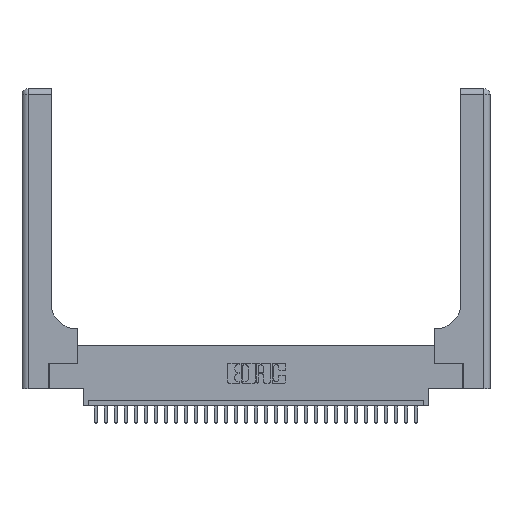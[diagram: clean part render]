
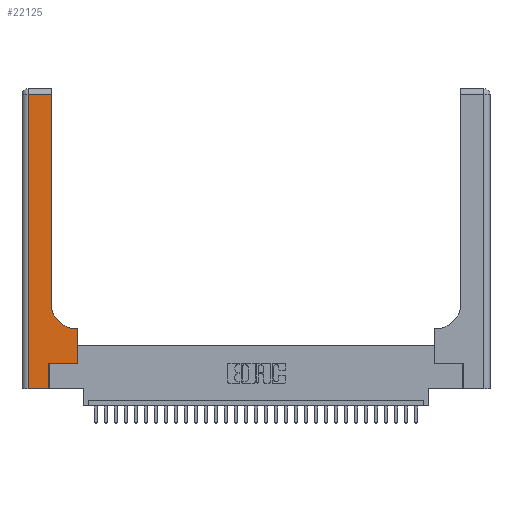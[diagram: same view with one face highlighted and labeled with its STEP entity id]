
A CAD part, top view. The second image highlights one B-rep face of the part: STEP entity #22125.
In plain terms, the highlighted planar face has unit normal (0, 0, 1).
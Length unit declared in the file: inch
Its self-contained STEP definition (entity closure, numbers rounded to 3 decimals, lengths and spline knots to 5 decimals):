
#57 = CARTESIAN_POINT ( 'NONE',  ( 0.269, 0.25, 0.37 ) ) ;
#70 = ORIENTED_EDGE ( 'NONE', *, *, #18516, .T. ) ;
#217 = DIRECTION ( 'NONE',  ( -1., 0., 0. ) ) ;
#860 = EDGE_CURVE ( 'NONE', #13966, #17433, #23793, .T. ) ;
#1548 = DIRECTION ( 'NONE',  ( 0., 1., 0. ) ) ;
#1826 = CARTESIAN_POINT ( 'NONE',  ( 0.5585, 0.6, 0.37 ) ) ;
#3278 = CARTESIAN_POINT ( 'NONE',  ( 0.2915, 0.85, 0.37 ) ) ;
#3948 = CARTESIAN_POINT ( 'NONE',  ( 0.5585, 0.25, 0.37 ) ) ;
#4366 = DIRECTION ( 'NONE',  ( 0., 1., 0. ) ) ;
#5008 = DIRECTION ( 'NONE',  ( 1., 0., 0. ) ) ;
#5168 = DIRECTION ( 'NONE',  ( 1., 0., 0. ) ) ;
#5256 = CARTESIAN_POINT ( 'NONE',  ( 0.2915, 0.6, 0.37 ) ) ;
#5613 = EDGE_LOOP ( 'NONE', ( #27200, #24012, #6091, #30341, #8297, #6652, #70, #12628, #13001 ) ) ;
#5722 = VERTEX_POINT ( 'NONE', #7020 ) ;
#6091 = ORIENTED_EDGE ( 'NONE', *, *, #7182, .T. ) ;
#6527 = VECTOR ( 'NONE', #7818, 39.37008 ) ;
#6652 = ORIENTED_EDGE ( 'NONE', *, *, #8832, .T. ) ;
#7020 = CARTESIAN_POINT ( 'NONE',  ( 0.2915, 2.94, 0.37 ) ) ;
#7182 = EDGE_CURVE ( 'NONE', #18581, #13966, #21991, .T. ) ;
#7818 = DIRECTION ( 'NONE',  ( -1., 0., 0. ) ) ;
#7889 = VECTOR ( 'NONE', #18866, 39.37008 ) ;
#8297 = ORIENTED_EDGE ( 'NONE', *, *, #11453, .T. ) ;
#8832 = EDGE_CURVE ( 'NONE', #22884, #28548, #8985, .T. ) ;
#8985 = LINE ( 'NONE', #16980, #14688 ) ;
#9966 = VERTEX_POINT ( 'NONE', #3278 ) ;
#10897 = VECTOR ( 'NONE', #1548, 39.37008 ) ;
#11356 = CARTESIAN_POINT ( 'NONE',  ( 0., 0., 0.37 ) ) ;
#11453 = EDGE_CURVE ( 'NONE', #17433, #22884, #26142, .T. ) ;
#12245 = CARTESIAN_POINT ( 'NONE',  ( 0.2915, 3., 0.37 ) ) ;
#12628 = ORIENTED_EDGE ( 'NONE', *, *, #26166, .T. ) ;
#13001 = ORIENTED_EDGE ( 'NONE', *, *, #15276, .T. ) ;
#13012 = VECTOR ( 'NONE', #26317, 39.37008 ) ;
#13784 = LINE ( 'NONE', #12245, #13012 ) ;
#13912 = CARTESIAN_POINT ( 'NONE',  ( 0.06, 0., 0.37 ) ) ;
#13966 = VERTEX_POINT ( 'NONE', #13912 ) ;
#14688 = VECTOR ( 'NONE', #5008, 39.37008 ) ;
#14939 = CIRCLE ( 'NONE', #19560, 0.25 ) ;
#15276 = EDGE_CURVE ( 'NONE', #17949, #9966, #14939, .T. ) ;
#16183 = CARTESIAN_POINT ( 'NONE',  ( 0.06, 2.94, 0.37 ) ) ;
#16445 = CARTESIAN_POINT ( 'NONE',  ( 0.269, 0., 0.37 ) ) ;
#16980 = CARTESIAN_POINT ( 'NONE',  ( 0.269, 0.25, 0.37 ) ) ;
#17208 = CARTESIAN_POINT ( 'NONE',  ( 0.269, 0., 0.37 ) ) ;
#17433 = VERTEX_POINT ( 'NONE', #17208 ) ;
#17570 = VERTEX_POINT ( 'NONE', #1826 ) ;
#17628 = AXIS2_PLACEMENT_3D ( 'NONE', #20672, #30501, #25644 ) ;
#17949 = VERTEX_POINT ( 'NONE', #23191 ) ;
#18255 = DIRECTION ( 'NONE',  ( 0., -1., 0. ) ) ;
#18516 = EDGE_CURVE ( 'NONE', #28548, #17570, #23756, .T. ) ;
#18581 = VERTEX_POINT ( 'NONE', #16183 ) ;
#18866 = DIRECTION ( 'NONE',  ( 1., 0., 0. ) ) ;
#19560 = AXIS2_PLACEMENT_3D ( 'NONE', #29234, #19966, #5168 ) ;
#19966 = DIRECTION ( 'NONE',  ( 0., 0., -1. ) ) ;
#20564 = LINE ( 'NONE', #26979, #6527 ) ;
#20672 = CARTESIAN_POINT ( 'NONE',  ( 0., 3., 0.37 ) ) ;
#20706 = LINE ( 'NONE', #5256, #23751 ) ;
#20761 = PLANE ( 'NONE',  #17628 ) ;
#20861 = VECTOR ( 'NONE', #4366, 39.37008 ) ;
#21036 = CARTESIAN_POINT ( 'NONE',  ( 0.5585, 0.25, 0.37 ) ) ;
#21991 = LINE ( 'NONE', #25460, #23880 ) ;
#22125 = ADVANCED_FACE ( 'NONE', ( #31197 ), #20761, .F. ) ;
#22884 = VERTEX_POINT ( 'NONE', #57 ) ;
#23191 = CARTESIAN_POINT ( 'NONE',  ( 0.5415, 0.6, 0.37 ) ) ;
#23751 = VECTOR ( 'NONE', #217, 39.37008 ) ;
#23756 = LINE ( 'NONE', #21036, #10897 ) ;
#23793 = LINE ( 'NONE', #11356, #7889 ) ;
#23880 = VECTOR ( 'NONE', #18255, 39.37008 ) ;
#24012 = ORIENTED_EDGE ( 'NONE', *, *, #30683, .T. ) ;
#25460 = CARTESIAN_POINT ( 'NONE',  ( 0.06, 3., 0.37 ) ) ;
#25644 = DIRECTION ( 'NONE',  ( -1., 0., 0. ) ) ;
#26142 = LINE ( 'NONE', #16445, #20861 ) ;
#26166 = EDGE_CURVE ( 'NONE', #17570, #17949, #20706, .T. ) ;
#26317 = DIRECTION ( 'NONE',  ( 0., 1., 0. ) ) ;
#26979 = CARTESIAN_POINT ( 'NONE',  ( 0., 2.94, 0.37 ) ) ;
#27200 = ORIENTED_EDGE ( 'NONE', *, *, #28108, .T. ) ;
#28108 = EDGE_CURVE ( 'NONE', #9966, #5722, #13784, .T. ) ;
#28548 = VERTEX_POINT ( 'NONE', #3948 ) ;
#29234 = CARTESIAN_POINT ( 'NONE',  ( 0.5415, 0.85, 0.37 ) ) ;
#30341 = ORIENTED_EDGE ( 'NONE', *, *, #860, .T. ) ;
#30501 = DIRECTION ( 'NONE',  ( 0., 0., -1. ) ) ;
#30683 = EDGE_CURVE ( 'NONE', #5722, #18581, #20564, .T. ) ;
#31197 = FACE_OUTER_BOUND ( 'NONE', #5613, .T. ) ;
